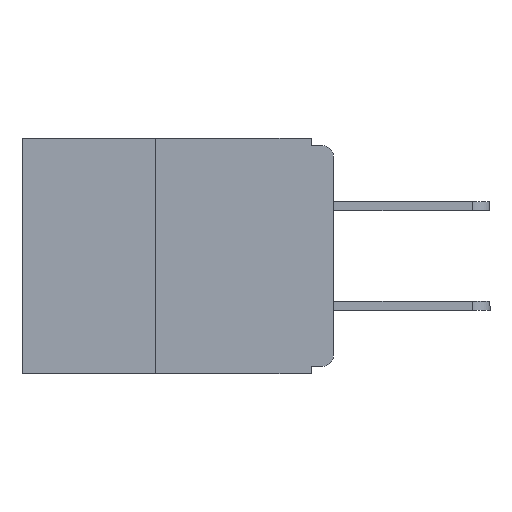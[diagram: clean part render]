
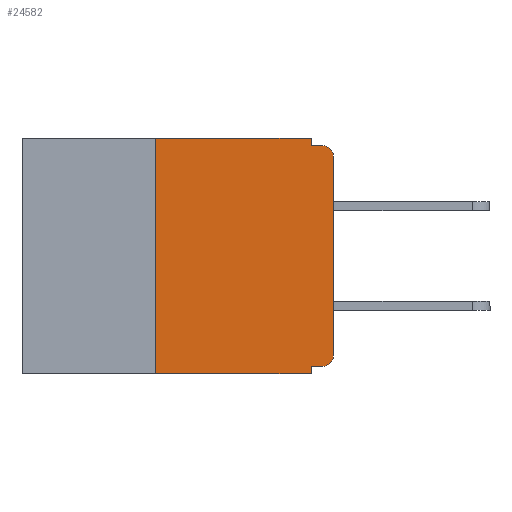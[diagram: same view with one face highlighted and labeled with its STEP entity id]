
A CAD part, left-side view. The second image highlights one B-rep face of the part: STEP entity #24582.
In plain terms, the highlighted planar face has unit normal (-1, 0, 0).
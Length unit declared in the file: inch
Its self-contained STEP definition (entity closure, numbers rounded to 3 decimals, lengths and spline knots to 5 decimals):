
#5 = ORIENTED_EDGE ( 'NONE', *, *, #13720, .T. ) ;
#231 = LINE ( 'NONE', #18632, #5431 ) ;
#258 = ORIENTED_EDGE ( 'NONE', *, *, #21671, .T. ) ;
#390 = AXIS2_PLACEMENT_3D ( 'NONE', #14856, #31432, #17233 ) ;
#1013 = CARTESIAN_POINT ( 'NONE',  ( 0., 0.031, -0.01 ) ) ;
#1088 = CARTESIAN_POINT ( 'NONE',  ( 0., 0.437, 0. ) ) ;
#1195 = CARTESIAN_POINT ( 'NONE',  ( 0., 0.031, -0.33 ) ) ;
#1312 = VERTEX_POINT ( 'NONE', #15495 ) ;
#1419 = DIRECTION ( 'NONE',  ( 0., 0., -1. ) ) ;
#1463 = LINE ( 'NONE', #6423, #26813 ) ;
#1822 = DIRECTION ( 'NONE',  ( 0., 0., -1. ) ) ;
#2562 = CARTESIAN_POINT ( 'NONE',  ( 0., 0.031, -0.32 ) ) ;
#3659 = ORIENTED_EDGE ( 'NONE', *, *, #26445, .T. ) ;
#4098 = VERTEX_POINT ( 'NONE', #2562 ) ;
#4156 = DIRECTION ( 'NONE',  ( 0., -1., 0. ) ) ;
#4161 = EDGE_CURVE ( 'NONE', #12831, #22134, #29837, .T. ) ;
#4563 = VECTOR ( 'NONE', #12679, 39.37008 ) ;
#5431 = VECTOR ( 'NONE', #25755, 39.37008 ) ;
#5451 = ORIENTED_EDGE ( 'NONE', *, *, #4161, .F. ) ;
#5849 = AXIS2_PLACEMENT_3D ( 'NONE', #1088, #13737, #30396 ) ;
#5868 = CARTESIAN_POINT ( 'NONE',  ( 0., 0.25, -0.33 ) ) ;
#5972 = ORIENTED_EDGE ( 'NONE', *, *, #15364, .F. ) ;
#6138 = CIRCLE ( 'NONE', #10526, 0.015 ) ;
#6423 = CARTESIAN_POINT ( 'NONE',  ( 0., 0.031, 0. ) ) ;
#6842 = CARTESIAN_POINT ( 'NONE',  ( 0., 0.031, -0.33 ) ) ;
#7070 = ORIENTED_EDGE ( 'NONE', *, *, #19431, .T. ) ;
#7765 = CARTESIAN_POINT ( 'NONE',  ( 0., 0.437, 0. ) ) ;
#7902 = EDGE_CURVE ( 'NONE', #21358, #8188, #19967, .T. ) ;
#8188 = VERTEX_POINT ( 'NONE', #29532 ) ;
#8955 = LINE ( 'NONE', #27104, #21207 ) ;
#9411 = CARTESIAN_POINT ( 'NONE',  ( 0., 0., -0.305 ) ) ;
#9578 = CIRCLE ( 'NONE', #390, 0.015 ) ;
#10416 = EDGE_CURVE ( 'NONE', #4098, #27665, #26198, .T. ) ;
#10526 = AXIS2_PLACEMENT_3D ( 'NONE', #30930, #16751, #1822 ) ;
#10741 = VECTOR ( 'NONE', #17546, 39.37008 ) ;
#11224 = ORIENTED_EDGE ( 'NONE', *, *, #31060, .F. ) ;
#12679 = DIRECTION ( 'NONE',  ( 0., 0., 1. ) ) ;
#12831 = VERTEX_POINT ( 'NONE', #17597 ) ;
#13642 = PLANE ( 'NONE',  #5849 ) ;
#13720 = EDGE_CURVE ( 'NONE', #25092, #27665, #231, .T. ) ;
#13737 = DIRECTION ( 'NONE',  ( 1., 0., 0. ) ) ;
#13788 = VECTOR ( 'NONE', #21728, 39.37008 ) ;
#14212 = CARTESIAN_POINT ( 'NONE',  ( 0., 0., -0.01 ) ) ;
#14509 = CARTESIAN_POINT ( 'NONE',  ( 0., 0.015, -0.32 ) ) ;
#14579 = LINE ( 'NONE', #24089, #13788 ) ;
#14856 = CARTESIAN_POINT ( 'NONE',  ( 0., 0.015, -0.305 ) ) ;
#15364 = EDGE_CURVE ( 'NONE', #25092, #12831, #16958, .T. ) ;
#15495 = CARTESIAN_POINT ( 'NONE',  ( 0., 0., -0.025 ) ) ;
#15853 = ORIENTED_EDGE ( 'NONE', *, *, #7902, .F. ) ;
#16360 = DIRECTION ( 'NONE',  ( 0., 0., -1. ) ) ;
#16751 = DIRECTION ( 'NONE',  ( -1., 0., 0. ) ) ;
#16958 = LINE ( 'NONE', #29319, #4563 ) ;
#17233 = DIRECTION ( 'NONE',  ( 0., 0., -1. ) ) ;
#17409 = ORIENTED_EDGE ( 'NONE', *, *, #10416, .F. ) ;
#17546 = DIRECTION ( 'NONE',  ( 0., -1., 0. ) ) ;
#17597 = CARTESIAN_POINT ( 'NONE',  ( 0., 0.25, 0. ) ) ;
#18438 = VECTOR ( 'NONE', #4156, 39.37008 ) ;
#18598 = EDGE_CURVE ( 'NONE', #22134, #21358, #1463, .T. ) ;
#18632 = CARTESIAN_POINT ( 'NONE',  ( 0., 0.437, -0.33 ) ) ;
#19431 = EDGE_CURVE ( 'NONE', #29797, #1312, #8955, .T. ) ;
#19852 = VECTOR ( 'NONE', #1419, 39.37008 ) ;
#19898 = VERTEX_POINT ( 'NONE', #14509 ) ;
#19967 = LINE ( 'NONE', #14212, #18438 ) ;
#20045 = DIRECTION ( 'NONE',  ( 0., 0., 1. ) ) ;
#21207 = VECTOR ( 'NONE', #20045, 39.37008 ) ;
#21358 = VERTEX_POINT ( 'NONE', #1013 ) ;
#21671 = EDGE_CURVE ( 'NONE', #19898, #29797, #9578, .T. ) ;
#21728 = DIRECTION ( 'NONE',  ( 0., 1., 0. ) ) ;
#22134 = VERTEX_POINT ( 'NONE', #26261 ) ;
#22347 = EDGE_LOOP ( 'NONE', ( #7070, #3659, #15853, #30331, #5451, #5972, #5, #17409, #11224, #258 ) ) ;
#23124 = FACE_OUTER_BOUND ( 'NONE', #22347, .T. ) ;
#24089 = CARTESIAN_POINT ( 'NONE',  ( 0., 0., -0.32 ) ) ;
#24582 = ADVANCED_FACE ( 'NONE', ( #23124 ), #13642, .F. ) ;
#25092 = VERTEX_POINT ( 'NONE', #5868 ) ;
#25755 = DIRECTION ( 'NONE',  ( 0., -1., 0. ) ) ;
#26198 = LINE ( 'NONE', #1195, #19852 ) ;
#26261 = CARTESIAN_POINT ( 'NONE',  ( 0., 0.031, 0. ) ) ;
#26445 = EDGE_CURVE ( 'NONE', #1312, #8188, #6138, .T. ) ;
#26813 = VECTOR ( 'NONE', #16360, 39.37008 ) ;
#27104 = CARTESIAN_POINT ( 'NONE',  ( 0., 0., 0. ) ) ;
#27665 = VERTEX_POINT ( 'NONE', #6842 ) ;
#29319 = CARTESIAN_POINT ( 'NONE',  ( 0., 0.25, -0.33 ) ) ;
#29532 = CARTESIAN_POINT ( 'NONE',  ( 0., 0.015, -0.01 ) ) ;
#29797 = VERTEX_POINT ( 'NONE', #9411 ) ;
#29837 = LINE ( 'NONE', #7765, #10741 ) ;
#30331 = ORIENTED_EDGE ( 'NONE', *, *, #18598, .F. ) ;
#30396 = DIRECTION ( 'NONE',  ( 0., 0., -1. ) ) ;
#30930 = CARTESIAN_POINT ( 'NONE',  ( 0., 0.015, -0.025 ) ) ;
#31060 = EDGE_CURVE ( 'NONE', #19898, #4098, #14579, .T. ) ;
#31432 = DIRECTION ( 'NONE',  ( -1., 0., 0. ) ) ;
